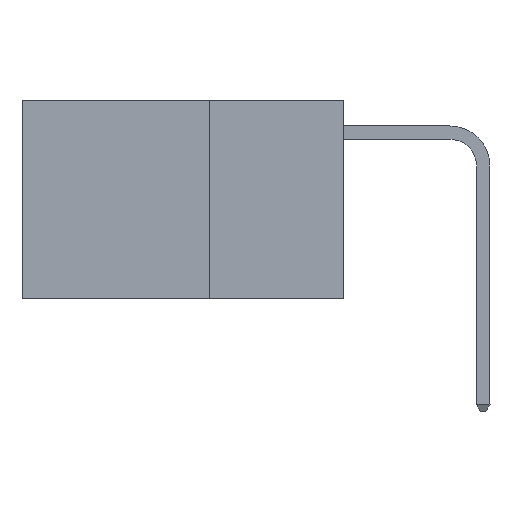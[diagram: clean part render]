
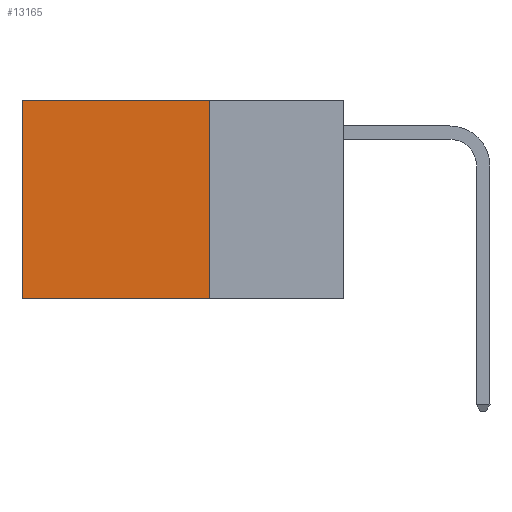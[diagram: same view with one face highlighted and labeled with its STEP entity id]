
A CAD part, left-side view. The second image highlights one B-rep face of the part: STEP entity #13165.
In plain terms, the highlighted planar face has unit normal (-1, 0, 0).
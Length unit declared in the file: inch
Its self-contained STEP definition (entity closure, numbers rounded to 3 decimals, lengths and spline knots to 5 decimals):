
#551 = EDGE_LOOP ( 'NONE', ( #17958, #15875, #20661, #2440 ) ) ;
#1028 = CARTESIAN_POINT ( 'NONE',  ( 0.2625, 0.6, 0. ) ) ;
#1460 = CARTESIAN_POINT ( 'NONE',  ( 0.2625, 0.6, -0.37 ) ) ;
#2440 = ORIENTED_EDGE ( 'NONE', *, *, #3016, .T. ) ;
#2923 = DIRECTION ( 'NONE',  ( 0., 1., 0. ) ) ;
#3016 = EDGE_CURVE ( 'NONE', #16783, #21590, #23946, .T. ) ;
#3339 = VECTOR ( 'NONE', #21821, 39.37008 ) ;
#3953 = CARTESIAN_POINT ( 'NONE',  ( 0.2625, 0.25, 0. ) ) ;
#4866 = VECTOR ( 'NONE', #14274, 39.37008 ) ;
#5503 = DIRECTION ( 'NONE',  ( 0., 0., -1. ) ) ;
#5856 = VERTEX_POINT ( 'NONE', #11419 ) ;
#5904 = DIRECTION ( 'NONE',  ( 1., 0., 0. ) ) ;
#6317 = LINE ( 'NONE', #14050, #3339 ) ;
#9360 = PLANE ( 'NONE',  #15837 ) ;
#11419 = CARTESIAN_POINT ( 'NONE',  ( 0.2625, 0.25, -0.37 ) ) ;
#13165 = ADVANCED_FACE ( 'NONE', ( #14904 ), #9360, .F. ) ;
#13901 = CARTESIAN_POINT ( 'NONE',  ( 0.2625, 0.25, 0. ) ) ;
#14050 = CARTESIAN_POINT ( 'NONE',  ( 0.2625, 0.6, 0. ) ) ;
#14274 = DIRECTION ( 'NONE',  ( 0., 1., 0. ) ) ;
#14904 = FACE_OUTER_BOUND ( 'NONE', #551, .T. ) ;
#15011 = LINE ( 'NONE', #17178, #18613 ) ;
#15837 = AXIS2_PLACEMENT_3D ( 'NONE', #19112, #5904, #23062 ) ;
#15875 = ORIENTED_EDGE ( 'NONE', *, *, #18133, .F. ) ;
#16563 = EDGE_CURVE ( 'NONE', #16783, #5856, #15011, .T. ) ;
#16783 = VERTEX_POINT ( 'NONE', #3953 ) ;
#17178 = CARTESIAN_POINT ( 'NONE',  ( 0.2625, 0.25, 0. ) ) ;
#17958 = ORIENTED_EDGE ( 'NONE', *, *, #19360, .T. ) ;
#18133 = EDGE_CURVE ( 'NONE', #5856, #20634, #22524, .T. ) ;
#18613 = VECTOR ( 'NONE', #5503, 39.37008 ) ;
#19112 = CARTESIAN_POINT ( 'NONE',  ( 0.2625, 0.25, 0. ) ) ;
#19360 = EDGE_CURVE ( 'NONE', #21590, #20634, #6317, .T. ) ;
#20597 = CARTESIAN_POINT ( 'NONE',  ( 0.2625, 0.25, -0.37 ) ) ;
#20634 = VERTEX_POINT ( 'NONE', #1460 ) ;
#20661 = ORIENTED_EDGE ( 'NONE', *, *, #16563, .F. ) ;
#21590 = VERTEX_POINT ( 'NONE', #1028 ) ;
#21821 = DIRECTION ( 'NONE',  ( 0., 0., -1. ) ) ;
#22524 = LINE ( 'NONE', #20597, #24665 ) ;
#23062 = DIRECTION ( 'NONE',  ( 0., 0., -1. ) ) ;
#23946 = LINE ( 'NONE', #13901, #4866 ) ;
#24665 = VECTOR ( 'NONE', #2923, 39.37008 ) ;
